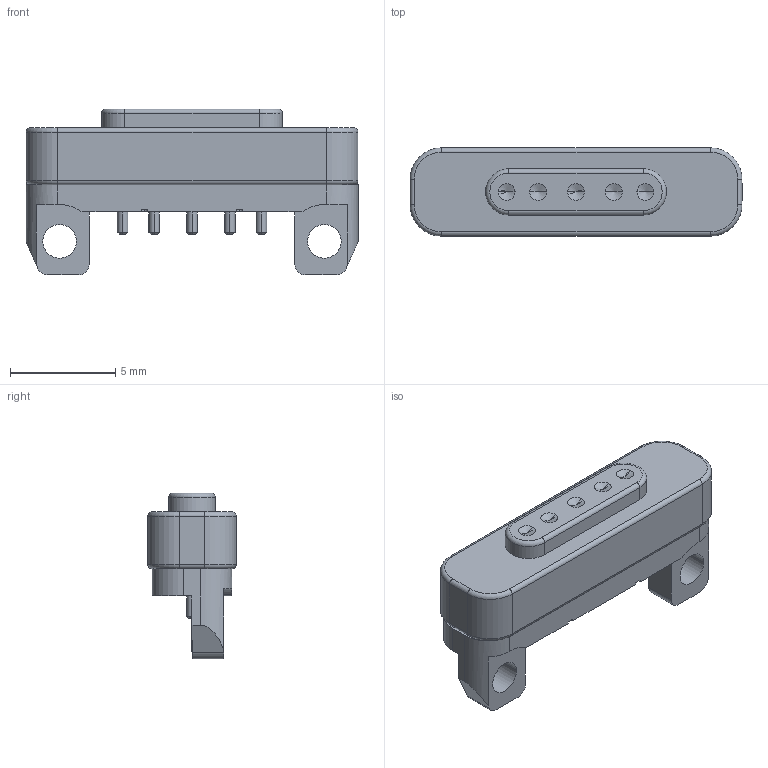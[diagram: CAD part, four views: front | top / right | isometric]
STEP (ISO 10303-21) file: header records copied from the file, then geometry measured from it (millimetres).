
FILE_DESCRIPTION (( 'STEP AP203' ), '1' );
FILE_NAME ('686-G0524250123.STEP', '2023-02-08T11:11:04', ( '' ), ( '' ), 'SwSTEP 2.0', 'SolidWorks 2020', '' );
FILE_SCHEMA (( 'CONFIG_CONTROL_DESIGN' ));
Length unit declared in the file: millimetre
Products named in the file (1): 686-G0524250123
Bounding box: 15.8 x 4.2 x 7.9 mm (x, y, z)
Surface area: 464.9 mm2 (no closed solid volume)
Topology: 0 solids, 7 shells, 154 faces, 395 edges, 251 vertices
Faces by surface type: cylinder 58, plane 58, cone 20, torus 18
Entity records: 4723 total; most frequent: DIRECTION 869, CARTESIAN_POINT 826, ORIENTED_EDGE 732, EDGE_CURVE 385, AXIS2_PLACEMENT_3D 331, VERTEX_POINT 251, LINE 207, VECTOR 207
